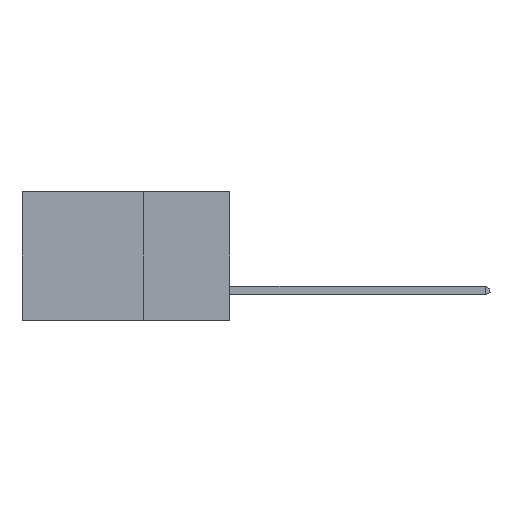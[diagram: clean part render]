
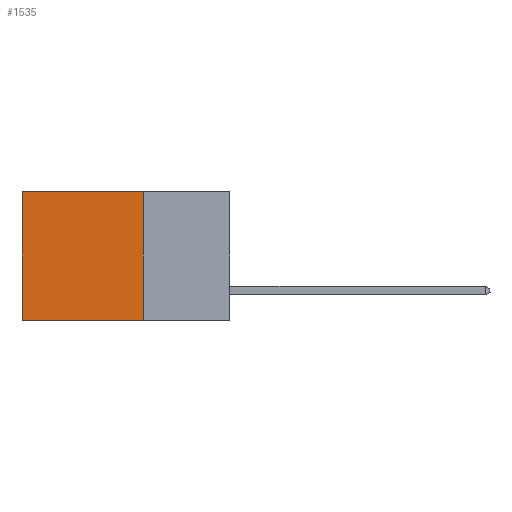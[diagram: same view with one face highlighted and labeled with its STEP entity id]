
A CAD part, left-side view. The second image highlights one B-rep face of the part: STEP entity #1535.
In plain terms, the highlighted planar face has unit normal (-1, 0, 0).
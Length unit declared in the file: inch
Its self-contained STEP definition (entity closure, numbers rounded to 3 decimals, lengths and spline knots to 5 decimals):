
#1072 = CARTESIAN_POINT ( 'NONE',  ( 0.298, 0.6, -0.37 ) ) ;
#1452 = VERTEX_POINT ( 'NONE', #7053 ) ;
#1519 = DIRECTION ( 'NONE',  ( 0., 1., 0. ) ) ;
#1535 = ADVANCED_FACE ( 'NONE', ( #6052 ), #24449, .F. ) ;
#1756 = DIRECTION ( 'NONE',  ( 0., 0., -1. ) ) ;
#2601 = ORIENTED_EDGE ( 'NONE', *, *, #21401, .T. ) ;
#2739 = EDGE_CURVE ( 'NONE', #6771, #1452, #8591, .T. ) ;
#2823 = DIRECTION ( 'NONE',  ( 0., 0., -1. ) ) ;
#3717 = AXIS2_PLACEMENT_3D ( 'NONE', #26972, #14398, #12034 ) ;
#4790 = VECTOR ( 'NONE', #1756, 39.37008 ) ;
#5058 = EDGE_LOOP ( 'NONE', ( #2601, #28598, #15414, #27934 ) ) ;
#5642 = VERTEX_POINT ( 'NONE', #8942 ) ;
#6052 = FACE_OUTER_BOUND ( 'NONE', #5058, .T. ) ;
#6771 = VERTEX_POINT ( 'NONE', #11834 ) ;
#7053 = CARTESIAN_POINT ( 'NONE',  ( 0.298, 0.6, 0. ) ) ;
#7153 = CARTESIAN_POINT ( 'NONE',  ( 0.298, 0.25, 0. ) ) ;
#8591 = LINE ( 'NONE', #7153, #28052 ) ;
#8942 = CARTESIAN_POINT ( 'NONE',  ( 0.298, 0.25, -0.37 ) ) ;
#9799 = VECTOR ( 'NONE', #2823, 39.37008 ) ;
#10082 = CARTESIAN_POINT ( 'NONE',  ( 0.298, 0.25, 0. ) ) ;
#11758 = CARTESIAN_POINT ( 'NONE',  ( 0.298, 0.6, 0. ) ) ;
#11834 = CARTESIAN_POINT ( 'NONE',  ( 0.298, 0.25, 0. ) ) ;
#12034 = DIRECTION ( 'NONE',  ( 0., 0., -1. ) ) ;
#14398 = DIRECTION ( 'NONE',  ( 1., 0., 0. ) ) ;
#14906 = EDGE_CURVE ( 'NONE', #6771, #5642, #24318, .T. ) ;
#15288 = VECTOR ( 'NONE', #1519, 39.37008 ) ;
#15414 = ORIENTED_EDGE ( 'NONE', *, *, #14906, .F. ) ;
#18627 = EDGE_CURVE ( 'NONE', #5642, #19571, #29379, .T. ) ;
#19571 = VERTEX_POINT ( 'NONE', #1072 ) ;
#20639 = CARTESIAN_POINT ( 'NONE',  ( 0.298, 0.25, -0.37 ) ) ;
#21401 = EDGE_CURVE ( 'NONE', #1452, #19571, #25404, .T. ) ;
#24318 = LINE ( 'NONE', #10082, #9799 ) ;
#24449 = PLANE ( 'NONE',  #3717 ) ;
#25404 = LINE ( 'NONE', #11758, #4790 ) ;
#26972 = CARTESIAN_POINT ( 'NONE',  ( 0.298, 0.25, 0. ) ) ;
#27934 = ORIENTED_EDGE ( 'NONE', *, *, #2739, .T. ) ;
#28052 = VECTOR ( 'NONE', #29090, 39.37008 ) ;
#28598 = ORIENTED_EDGE ( 'NONE', *, *, #18627, .F. ) ;
#29090 = DIRECTION ( 'NONE',  ( 0., 1., 0. ) ) ;
#29379 = LINE ( 'NONE', #20639, #15288 ) ;
